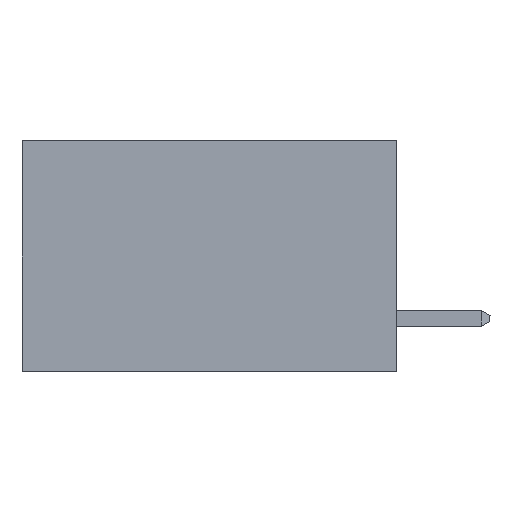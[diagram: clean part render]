
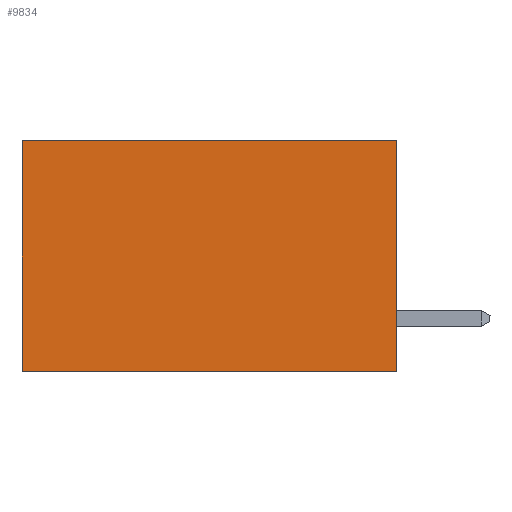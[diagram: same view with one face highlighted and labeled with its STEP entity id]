
A CAD part, left-side view. The second image highlights one B-rep face of the part: STEP entity #9834.
In plain terms, the highlighted planar face has unit normal (-1, 0, 0).
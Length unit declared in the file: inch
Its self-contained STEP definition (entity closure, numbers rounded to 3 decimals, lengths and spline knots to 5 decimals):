
#476 = LINE ( 'NONE', #18386, #3001 ) ;
#811 = CARTESIAN_POINT ( 'NONE',  ( 0.2615, 0.6, -0.37 ) ) ;
#1360 = VERTEX_POINT ( 'NONE', #13373 ) ;
#1397 = DIRECTION ( 'NONE',  ( 0., 1., 0. ) ) ;
#1956 = VERTEX_POINT ( 'NONE', #16639 ) ;
#2222 = VECTOR ( 'NONE', #17119, 39.37008 ) ;
#2984 = VERTEX_POINT ( 'NONE', #811 ) ;
#3001 = VECTOR ( 'NONE', #9687, 39.37008 ) ;
#4935 = CARTESIAN_POINT ( 'NONE',  ( 0.2615, 0.6, -0.37 ) ) ;
#5059 = EDGE_CURVE ( 'NONE', #1360, #2984, #13507, .T. ) ;
#5392 = DIRECTION ( 'NONE',  ( 0., 0., -1. ) ) ;
#5938 = FACE_OUTER_BOUND ( 'NONE', #17613, .T. ) ;
#6161 = CARTESIAN_POINT ( 'NONE',  ( 0.2615, 0., 0. ) ) ;
#7103 = LINE ( 'NONE', #13627, #2222 ) ;
#8402 = ORIENTED_EDGE ( 'NONE', *, *, #21408, .F. ) ;
#8835 = VECTOR ( 'NONE', #5392, 39.37008 ) ;
#9687 = DIRECTION ( 'NONE',  ( 0., 1., 0. ) ) ;
#9834 = ADVANCED_FACE ( 'NONE', ( #5938 ), #13047, .F. ) ;
#10673 = CARTESIAN_POINT ( 'NONE',  ( 0.2615, 0., 0. ) ) ;
#10787 = VECTOR ( 'NONE', #1397, 39.37008 ) ;
#13021 = DIRECTION ( 'NONE',  ( 0., 0., -1. ) ) ;
#13042 = DIRECTION ( 'NONE',  ( 1., 0., 0. ) ) ;
#13047 = PLANE ( 'NONE',  #17788 ) ;
#13115 = CARTESIAN_POINT ( 'NONE',  ( 0.2615, 0., -0.37 ) ) ;
#13257 = EDGE_CURVE ( 'NONE', #16120, #1360, #15444, .T. ) ;
#13373 = CARTESIAN_POINT ( 'NONE',  ( 0.2615, 0.6, 0. ) ) ;
#13507 = LINE ( 'NONE', #4935, #8835 ) ;
#13627 = CARTESIAN_POINT ( 'NONE',  ( 0.2615, 0., -0.37 ) ) ;
#14296 = ORIENTED_EDGE ( 'NONE', *, *, #13257, .T. ) ;
#14665 = EDGE_CURVE ( 'NONE', #16120, #1956, #7103, .T. ) ;
#15444 = LINE ( 'NONE', #10673, #10787 ) ;
#15579 = ORIENTED_EDGE ( 'NONE', *, *, #5059, .T. ) ;
#16120 = VERTEX_POINT ( 'NONE', #6161 ) ;
#16401 = ORIENTED_EDGE ( 'NONE', *, *, #14665, .F. ) ;
#16639 = CARTESIAN_POINT ( 'NONE',  ( 0.2615, 0., -0.37 ) ) ;
#17119 = DIRECTION ( 'NONE',  ( 0., 0., -1. ) ) ;
#17613 = EDGE_LOOP ( 'NONE', ( #15579, #8402, #16401, #14296 ) ) ;
#17788 = AXIS2_PLACEMENT_3D ( 'NONE', #13115, #13042, #13021 ) ;
#18386 = CARTESIAN_POINT ( 'NONE',  ( 0.2615, 0., -0.37 ) ) ;
#21408 = EDGE_CURVE ( 'NONE', #1956, #2984, #476, .T. ) ;
